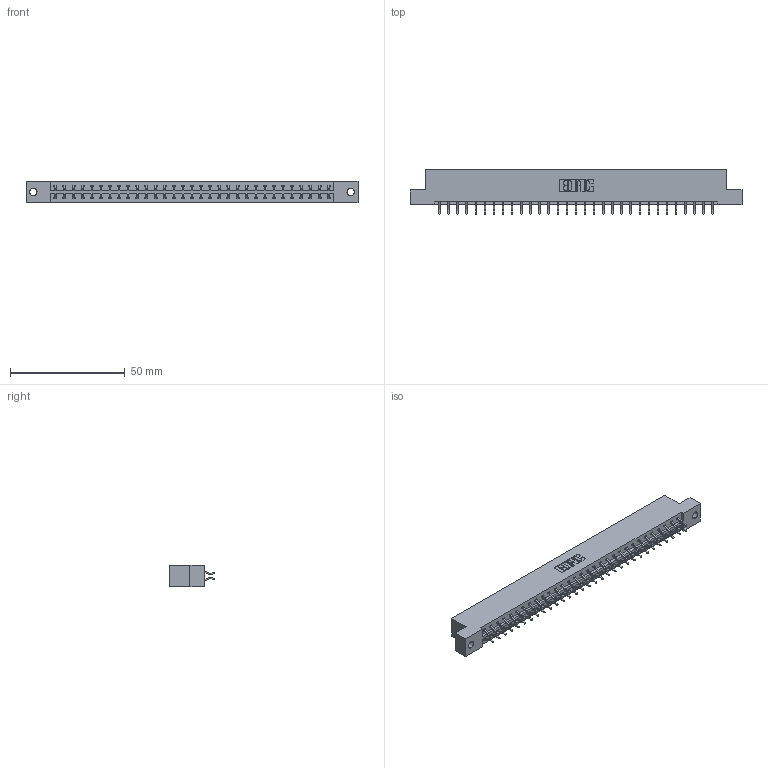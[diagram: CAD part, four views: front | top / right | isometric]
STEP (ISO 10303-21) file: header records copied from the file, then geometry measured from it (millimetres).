
FILE_DESCRIPTION (( 'STEP AP203' ), '1' );
FILE_NAME ('833-062-556-202.STEP', '2020-06-05T06:06:32', ( '' ), ( '' ), 'SwSTEP 2.0', 'SolidWorks 2020', '' );
FILE_SCHEMA (( 'CONFIG_CONTROL_DESIGN' ));
Length unit declared in the file: inch
Products named in the file (3): 833-062-556-202; 345-292-001_556 Tail; 833 Part_Flush - .128 Dia
Assembly tree (63 placements, depth 2):
  833-062-556-202
    833 Part_Flush - .128 Dia
    345-292-001_556 Tail  x62
Bounding box: 144.37 x 19.57 x 9.4 mm (x, y, z)
Volume: 14597.7 mm3; surface area: 16805.4 mm2
Topology: 63 solids, 63 shells, 3710 faces, 11037 edges, 7274 vertices
Faces by surface type: plane 2550, cylinder 1160
Entity records: 21589 total; most frequent: CARTESIAN_POINT 3606, ORIENTED_EDGE 3530, DIRECTION 3089, EDGE_CURVE 1765, VECTOR 1629, LINE 1629, VERTEX_POINT 1174, AXIS2_PLACEMENT_3D 730
